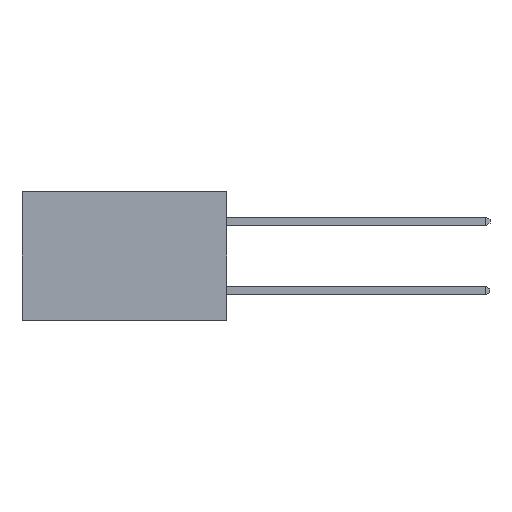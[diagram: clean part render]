
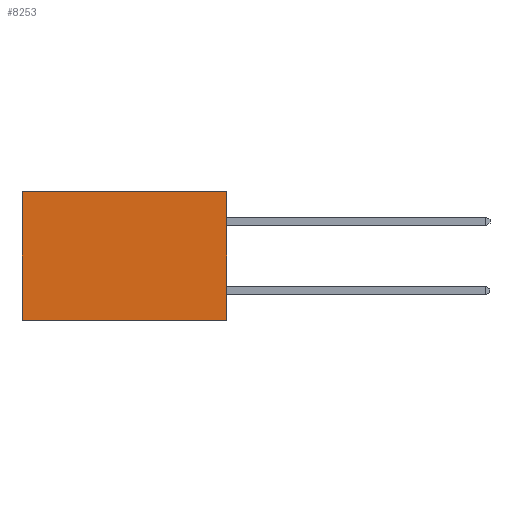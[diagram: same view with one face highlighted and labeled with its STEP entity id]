
A CAD part, left-side view. The second image highlights one B-rep face of the part: STEP entity #8253.
In plain terms, the highlighted planar face has unit normal (-1, 0, 0).
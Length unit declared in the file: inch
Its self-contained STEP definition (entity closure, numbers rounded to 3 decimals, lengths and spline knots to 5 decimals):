
#369 = LINE ( 'NONE', #11347, #10340 ) ;
#721 = CARTESIAN_POINT ( 'NONE',  ( 0.277, 0., -0.37 ) ) ;
#1171 = DIRECTION ( 'NONE',  ( 0., 0., -1. ) ) ;
#1581 = LINE ( 'NONE', #3063, #11311 ) ;
#1984 = DIRECTION ( 'NONE',  ( 0., 0., -1. ) ) ;
#2370 = ORIENTED_EDGE ( 'NONE', *, *, #2980, .F. ) ;
#2937 = CARTESIAN_POINT ( 'NONE',  ( 0.277, 0., 0. ) ) ;
#2980 = EDGE_CURVE ( 'NONE', #4171, #7397, #1581, .T. ) ;
#2996 = EDGE_CURVE ( 'NONE', #7397, #7659, #11046, .T. ) ;
#3063 = CARTESIAN_POINT ( 'NONE',  ( 0.277, 0., -0.37 ) ) ;
#3483 = DIRECTION ( 'NONE',  ( 0., 0., -1. ) ) ;
#3786 = VECTOR ( 'NONE', #3483, 39.37008 ) ;
#4171 = VERTEX_POINT ( 'NONE', #2937 ) ;
#4475 = CARTESIAN_POINT ( 'NONE',  ( 0.277, 0., -0.37 ) ) ;
#4652 = EDGE_LOOP ( 'NONE', ( #4717, #7395, #2370, #5031 ) ) ;
#4717 = ORIENTED_EDGE ( 'NONE', *, *, #6665, .T. ) ;
#4744 = FACE_OUTER_BOUND ( 'NONE', #4652, .T. ) ;
#5031 = ORIENTED_EDGE ( 'NONE', *, *, #6846, .T. ) ;
#5998 = CARTESIAN_POINT ( 'NONE',  ( 0.277, 0., -0.37 ) ) ;
#6574 = LINE ( 'NONE', #7537, #3786 ) ;
#6665 = EDGE_CURVE ( 'NONE', #11457, #7659, #6574, .T. ) ;
#6846 = EDGE_CURVE ( 'NONE', #4171, #11457, #369, .T. ) ;
#7395 = ORIENTED_EDGE ( 'NONE', *, *, #2996, .F. ) ;
#7397 = VERTEX_POINT ( 'NONE', #4475 ) ;
#7537 = CARTESIAN_POINT ( 'NONE',  ( 0.277, 0.59, -0.37 ) ) ;
#7659 = VERTEX_POINT ( 'NONE', #8560 ) ;
#7934 = DIRECTION ( 'NONE',  ( 1., 0., 0. ) ) ;
#8253 = ADVANCED_FACE ( 'NONE', ( #4744 ), #12172, .F. ) ;
#8560 = CARTESIAN_POINT ( 'NONE',  ( 0.277, 0.59, -0.37 ) ) ;
#8797 = VECTOR ( 'NONE', #9005, 39.37008 ) ;
#9005 = DIRECTION ( 'NONE',  ( 0., 1., 0. ) ) ;
#9315 = CARTESIAN_POINT ( 'NONE',  ( 0.277, 0.59, 0. ) ) ;
#10340 = VECTOR ( 'NONE', #11379, 39.37008 ) ;
#11046 = LINE ( 'NONE', #721, #8797 ) ;
#11311 = VECTOR ( 'NONE', #1171, 39.37008 ) ;
#11347 = CARTESIAN_POINT ( 'NONE',  ( 0.277, 0., 0. ) ) ;
#11379 = DIRECTION ( 'NONE',  ( 0., 1., 0. ) ) ;
#11455 = AXIS2_PLACEMENT_3D ( 'NONE', #5998, #7934, #1984 ) ;
#11457 = VERTEX_POINT ( 'NONE', #9315 ) ;
#12172 = PLANE ( 'NONE',  #11455 ) ;
